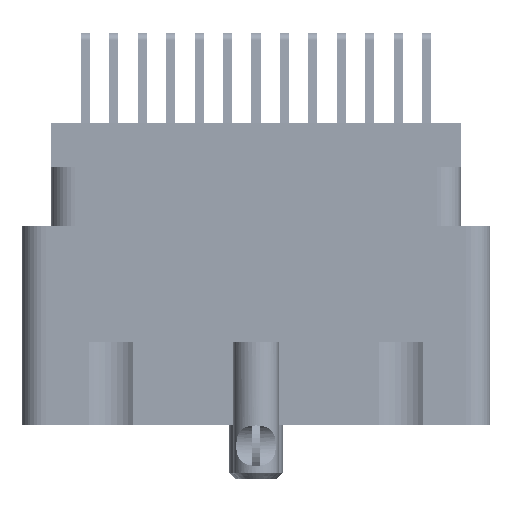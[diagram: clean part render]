
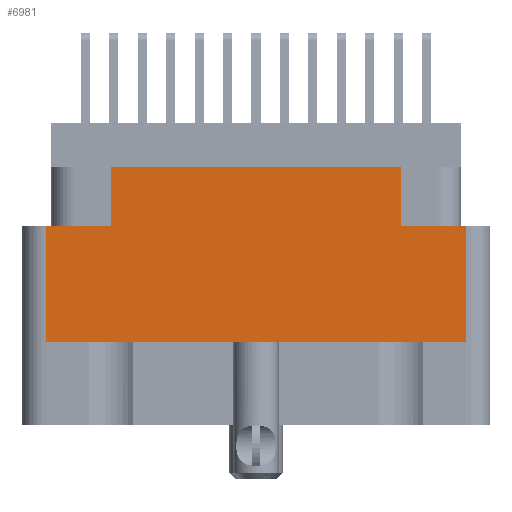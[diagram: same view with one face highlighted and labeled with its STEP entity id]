
A CAD part, left-side view. The second image highlights one B-rep face of the part: STEP entity #6981.
In plain terms, the highlighted planar face has unit normal (-1, 0, 0).
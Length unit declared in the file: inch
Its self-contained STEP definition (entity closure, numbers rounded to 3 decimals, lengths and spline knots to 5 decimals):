
#854 = VERTEX_POINT ( 'NONE', #30737 ) ;
#4428 = FACE_OUTER_BOUND ( 'NONE', #22119, .T. ) ;
#4840 = LINE ( 'NONE', #30013, #76633 ) ;
#5227 = DIRECTION ( 'NONE',  ( 0., 0., 1. ) ) ;
#6246 = CARTESIAN_POINT ( 'NONE',  ( -1.359, -0.555, -0.578 ) ) ;
#6981 = ADVANCED_FACE ( 'NONE', ( #4428 ), #49001, .T. ) ;
#7190 = DIRECTION ( 'NONE',  ( 0., -1., 0. ) ) ;
#9219 = VECTOR ( 'NONE', #45079, 39.37008 ) ;
#12135 = EDGE_CURVE ( 'NONE', #50100, #46477, #26081, .T. ) ;
#13002 = DIRECTION ( 'NONE',  ( 0., 0., 1. ) ) ;
#13470 = EDGE_CURVE ( 'NONE', #46008, #854, #50046, .T. ) ;
#13780 = LINE ( 'NONE', #77352, #78536 ) ;
#14105 = CARTESIAN_POINT ( 'NONE',  ( -1.359, 0.617, -0.117 ) ) ;
#14904 = VECTOR ( 'NONE', #55699, 39.37008 ) ;
#15495 = VERTEX_POINT ( 'NONE', #41904 ) ;
#17710 = CARTESIAN_POINT ( 'NONE',  ( -1.359, -0.555, -0.798 ) ) ;
#18684 = DIRECTION ( 'NONE',  ( 0., 0., -1. ) ) ;
#19156 = CARTESIAN_POINT ( 'NONE',  ( -1.359, 0.3825, -0.274 ) ) ;
#19903 = CARTESIAN_POINT ( 'NONE',  ( -1.359, -0.3825, -0.274 ) ) ;
#20530 = CARTESIAN_POINT ( 'NONE',  ( -1.359, -0.555, -0.274 ) ) ;
#22119 = EDGE_LOOP ( 'NONE', ( #40335, #73487, #29735, #79067, #76938, #33512, #76774, #54273 ) ) ;
#23070 = CARTESIAN_POINT ( 'NONE',  ( -1.359, 0.555, -0.274 ) ) ;
#25298 = CARTESIAN_POINT ( 'NONE',  ( -1.359, 0., -0.274 ) ) ;
#25559 = VERTEX_POINT ( 'NONE', #6246 ) ;
#26081 = LINE ( 'NONE', #19903, #9219 ) ;
#26215 = LINE ( 'NONE', #33244, #73435 ) ;
#28757 = AXIS2_PLACEMENT_3D ( 'NONE', #73384, #43191, #5227 ) ;
#29735 = ORIENTED_EDGE ( 'NONE', *, *, #30650, .T. ) ;
#30013 = CARTESIAN_POINT ( 'NONE',  ( -1.359, 0., -0.578 ) ) ;
#30650 = EDGE_CURVE ( 'NONE', #854, #25559, #4840, .T. ) ;
#30737 = CARTESIAN_POINT ( 'NONE',  ( -1.359, 0.555, -0.578 ) ) ;
#31305 = LINE ( 'NONE', #17710, #14904 ) ;
#31664 = DIRECTION ( 'NONE',  ( 0., -1., 0. ) ) ;
#33244 = CARTESIAN_POINT ( 'NONE',  ( -1.359, 0.3825, -0.274 ) ) ;
#33512 = ORIENTED_EDGE ( 'NONE', *, *, #12135, .T. ) ;
#37829 = EDGE_CURVE ( 'NONE', #25559, #46197, #31305, .T. ) ;
#38901 = DIRECTION ( 'NONE',  ( 0., -1., 0. ) ) ;
#39897 = EDGE_CURVE ( 'NONE', #15495, #46477, #45095, .T. ) ;
#40335 = ORIENTED_EDGE ( 'NONE', *, *, #80573, .F. ) ;
#41904 = CARTESIAN_POINT ( 'NONE',  ( -1.359, 0.3825, -0.117 ) ) ;
#43191 = DIRECTION ( 'NONE',  ( -1., 0., 0. ) ) ;
#43597 = VECTOR ( 'NONE', #63247, 39.37008 ) ;
#45079 = DIRECTION ( 'NONE',  ( 0., 0., 1. ) ) ;
#45095 = LINE ( 'NONE', #14105, #67675 ) ;
#45468 = CARTESIAN_POINT ( 'NONE',  ( -1.359, 0.555, -0.798 ) ) ;
#46008 = VERTEX_POINT ( 'NONE', #23070 ) ;
#46197 = VERTEX_POINT ( 'NONE', #20530 ) ;
#46477 = VERTEX_POINT ( 'NONE', #53923 ) ;
#47228 = VECTOR ( 'NONE', #18684, 39.37008 ) ;
#49001 = PLANE ( 'NONE',  #28757 ) ;
#50046 = LINE ( 'NONE', #45468, #47228 ) ;
#50100 = VERTEX_POINT ( 'NONE', #67601 ) ;
#51500 = EDGE_CURVE ( 'NONE', #50100, #46197, #13780, .T. ) ;
#53923 = CARTESIAN_POINT ( 'NONE',  ( -1.359, -0.3825, -0.117 ) ) ;
#54273 = ORIENTED_EDGE ( 'NONE', *, *, #60489, .F. ) ;
#55699 = DIRECTION ( 'NONE',  ( 0., 0., 1. ) ) ;
#60489 = EDGE_CURVE ( 'NONE', #76544, #15495, #26215, .T. ) ;
#63247 = DIRECTION ( 'NONE',  ( 0., -1., 0. ) ) ;
#67601 = CARTESIAN_POINT ( 'NONE',  ( -1.359, -0.3825, -0.274 ) ) ;
#67675 = VECTOR ( 'NONE', #38901, 39.37008 ) ;
#73384 = CARTESIAN_POINT ( 'NONE',  ( -1.359, -0.617, -0.798 ) ) ;
#73435 = VECTOR ( 'NONE', #13002, 39.37008 ) ;
#73487 = ORIENTED_EDGE ( 'NONE', *, *, #13470, .T. ) ;
#75685 = LINE ( 'NONE', #25298, #43597 ) ;
#76544 = VERTEX_POINT ( 'NONE', #19156 ) ;
#76633 = VECTOR ( 'NONE', #31664, 39.37008 ) ;
#76774 = ORIENTED_EDGE ( 'NONE', *, *, #39897, .F. ) ;
#76938 = ORIENTED_EDGE ( 'NONE', *, *, #51500, .F. ) ;
#77352 = CARTESIAN_POINT ( 'NONE',  ( -1.359, 0., -0.274 ) ) ;
#78536 = VECTOR ( 'NONE', #7190, 39.37008 ) ;
#79067 = ORIENTED_EDGE ( 'NONE', *, *, #37829, .T. ) ;
#80573 = EDGE_CURVE ( 'NONE', #46008, #76544, #75685, .T. ) ;
